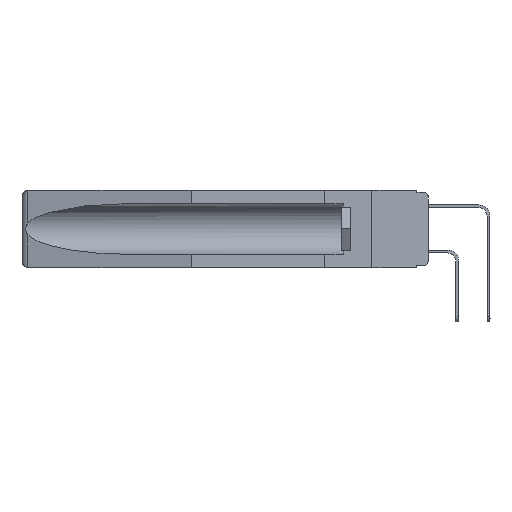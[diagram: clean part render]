
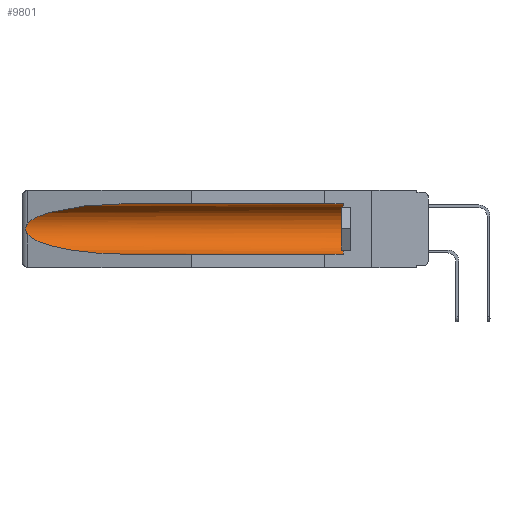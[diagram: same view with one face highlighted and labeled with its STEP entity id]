
A CAD part, left-side view. The second image highlights one B-rep face of the part: STEP entity #9801.
In plain terms, the highlighted cylindrical face has radius 2.857 mm (diameter 5.715 mm), a partial arc.
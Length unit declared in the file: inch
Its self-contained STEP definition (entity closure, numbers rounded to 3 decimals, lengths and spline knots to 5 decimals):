
#603 = VECTOR ( 'NONE', #15078, 39.37008 ) ;
#1464 = CARTESIAN_POINT ( 'NONE',  ( 0.155, 0.126, -0.1715 ) ) ;
#2020 = CARTESIAN_POINT ( 'NONE',  ( 0.26654, 1.53092, -0.15636 ) ) ;
#2167 = CARTESIAN_POINT ( 'NONE',  ( 0.155, -0.30754, -0.284 ) ) ;
#2761 = CARTESIAN_POINT ( 'NONE',  ( 0.155, -0.30754, -0.059 ) ) ;
#2980 = CARTESIAN_POINT ( 'NONE',  ( 0.21114, 1.30732, -0.284 ) ) ;
#4954 = LINE ( 'NONE', #2761, #603 ) ;
#5275 = ORIENTED_EDGE ( 'NONE', *, *, #6427, .T. ) ;
#5695 = CARTESIAN_POINT ( 'NONE',  ( 0.25451, 1.48313, -0.09465 ) ) ;
#5704 = DIRECTION ( 'NONE',  ( 0., -1., 0. ) ) ;
#6116 = CARTESIAN_POINT ( 'NONE',  ( 0.2675, 1.53308, -0.17534 ) ) ;
#6427 = EDGE_CURVE ( 'NONE', #25830, #20393, #13431, .T. ) ;
#6483 = CARTESIAN_POINT ( 'NONE',  ( 0.26537, 1.52718, -0.19328 ) ) ;
#6533 = ORIENTED_EDGE ( 'NONE', *, *, #13037, .T. ) ;
#6636 = DIRECTION ( 'NONE',  ( 0., 0., 1. ) ) ;
#7256 = DIRECTION ( 'NONE',  ( 0., 1., 0. ) ) ;
#7259 = CARTESIAN_POINT ( 'NONE',  ( 0.155, 1.07973, -0.284 ) ) ;
#7905 = EDGE_CURVE ( 'NONE', #25830, #11108, #22348, .T. ) ;
#8157 = CARTESIAN_POINT ( 'NONE',  ( 0.26655, 1.53094, -0.18657 ) ) ;
#8222 = EDGE_LOOP ( 'NONE', ( #6533, #8251, #23166, #24774, #5275, #18870 ) ) ;
#8251 = ORIENTED_EDGE ( 'NONE', *, *, #11870, .T. ) ;
#8570 = CARTESIAN_POINT ( 'NONE',  ( 0.26597, 1.52961, -0.15275 ) ) ;
#9385 = B_SPLINE_CURVE_WITH_KNOTS ( 'NONE', 3,
 ( #12184, #8570, #2020, #24597, #20548, #6116, #20284, #8157, #10313, #20409 ),
 .UNSPECIFIED., .F., .F.,
 ( 4, 2, 2, 2, 4 ),
 ( 0., 0.00029, 0.00058, 0.00087, 0.00117 ),
 .UNSPECIFIED. ) ;
#9522 = CARTESIAN_POINT ( 'NONE',  ( 0.155, 0.126, -0.284 ) ) ;
#9801 = ADVANCED_FACE ( 'NONE', ( #15190 ), #25724, .F. ) ;
#10194 =( BOUNDED_CURVE ( )  B_SPLINE_CURVE ( 3, ( #22031, #15683, #5695, #24189 ),
 .UNSPECIFIED., .F., .T. ) 
 B_SPLINE_CURVE_WITH_KNOTS ( ( 4, 4 ),
 ( 4.71239, 6.08839 ),
 .UNSPECIFIED. ) 
 CURVE ( )  GEOMETRIC_REPRESENTATION_ITEM ( )  RATIONAL_B_SPLINE_CURVE ( ( 1., 0.848, 0.848, 1. ) ) 
 REPRESENTATION_ITEM ( '' )  );
#10313 = CARTESIAN_POINT ( 'NONE',  ( 0.26597, 1.5296, -0.19026 ) ) ;
#10737 = CARTESIAN_POINT ( 'NONE',  ( 0.26537, 1.52718, -0.14972 ) ) ;
#10738 = CARTESIAN_POINT ( 'NONE',  ( 0.155, 1.07973, -0.284 ) ) ;
#10996 = CARTESIAN_POINT ( 'NONE',  ( 0.25451, 1.48313, -0.24835 ) ) ;
#11108 = VERTEX_POINT ( 'NONE', #7259 ) ;
#11786 = AXIS2_PLACEMENT_3D ( 'NONE', #13174, #7256, #15464 ) ;
#11870 = EDGE_CURVE ( 'NONE', #19517, #12542, #9385, .T. ) ;
#12184 = CARTESIAN_POINT ( 'NONE',  ( 0.26537, 1.52718, -0.14972 ) ) ;
#12542 = VERTEX_POINT ( 'NONE', #6483 ) ;
#12985 = AXIS2_PLACEMENT_3D ( 'NONE', #1464, #5704, #6636 ) ;
#13037 = EDGE_CURVE ( 'NONE', #22188, #19517, #10194, .T. ) ;
#13174 = CARTESIAN_POINT ( 'NONE',  ( 0.155, -0.30754, -0.1715 ) ) ;
#13279 = CARTESIAN_POINT ( 'NONE',  ( 0.26537, 1.52718, -0.19328 ) ) ;
#13431 = CIRCLE ( 'NONE', #12985, 0.1125 ) ;
#13524 = CARTESIAN_POINT ( 'NONE',  ( 0.155, 1.07973, -0.059 ) ) ;
#15078 = DIRECTION ( 'NONE',  ( 0., 1., 0. ) ) ;
#15190 = FACE_OUTER_BOUND ( 'NONE', #8222, .T. ) ;
#15464 = DIRECTION ( 'NONE',  ( 0., 0., 1. ) ) ;
#15683 = CARTESIAN_POINT ( 'NONE',  ( 0.21114, 1.30732, -0.059 ) ) ;
#16259 = DIRECTION ( 'NONE',  ( 0., 1., 0. ) ) ;
#18185 = VECTOR ( 'NONE', #16259, 39.37008 ) ;
#18870 = ORIENTED_EDGE ( 'NONE', *, *, #24368, .T. ) ;
#19517 = VERTEX_POINT ( 'NONE', #10737 ) ;
#20284 = CARTESIAN_POINT ( 'NONE',  ( 0.2673, 1.53269, -0.17917 ) ) ;
#20393 = VERTEX_POINT ( 'NONE', #20746 ) ;
#20409 = CARTESIAN_POINT ( 'NONE',  ( 0.26537, 1.52718, -0.19328 ) ) ;
#20548 = CARTESIAN_POINT ( 'NONE',  ( 0.2675, 1.53308, -0.16763 ) ) ;
#20746 = CARTESIAN_POINT ( 'NONE',  ( 0.155, 0.126, -0.059 ) ) ;
#22031 = CARTESIAN_POINT ( 'NONE',  ( 0.155, 1.07973, -0.059 ) ) ;
#22188 = VERTEX_POINT ( 'NONE', #13524 ) ;
#22348 = LINE ( 'NONE', #2167, #18185 ) ;
#23166 = ORIENTED_EDGE ( 'NONE', *, *, #25747, .T. ) ;
#24189 = CARTESIAN_POINT ( 'NONE',  ( 0.26537, 1.52718, -0.14972 ) ) ;
#24368 = EDGE_CURVE ( 'NONE', #20393, #22188, #4954, .T. ) ;
#24597 = CARTESIAN_POINT ( 'NONE',  ( 0.2673, 1.5327, -0.16383 ) ) ;
#24774 = ORIENTED_EDGE ( 'NONE', *, *, #7905, .F. ) ;
#24997 =( BOUNDED_CURVE ( )  B_SPLINE_CURVE ( 3, ( #13279, #10996, #2980, #10738 ),
 .UNSPECIFIED., .F., .T. ) 
 B_SPLINE_CURVE_WITH_KNOTS ( ( 4, 4 ),
 ( 0.1948, 1.5708 ),
 .UNSPECIFIED. ) 
 CURVE ( )  GEOMETRIC_REPRESENTATION_ITEM ( )  RATIONAL_B_SPLINE_CURVE ( ( 1., 0.848, 0.848, 1. ) ) 
 REPRESENTATION_ITEM ( '' )  );
#25724 = CYLINDRICAL_SURFACE ( 'NONE', #11786, 0.1125 ) ;
#25747 = EDGE_CURVE ( 'NONE', #12542, #11108, #24997, .T. ) ;
#25830 = VERTEX_POINT ( 'NONE', #9522 ) ;
